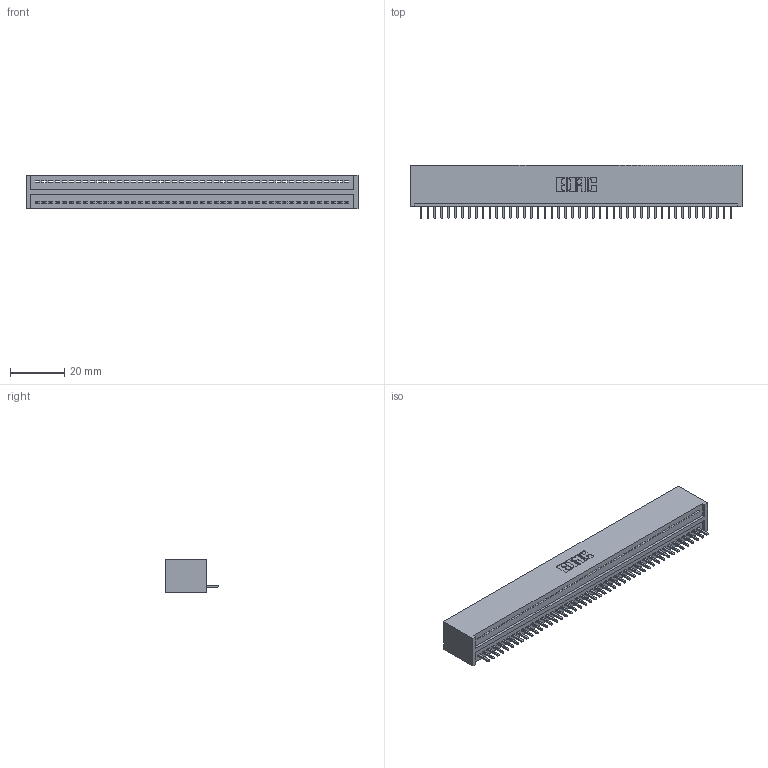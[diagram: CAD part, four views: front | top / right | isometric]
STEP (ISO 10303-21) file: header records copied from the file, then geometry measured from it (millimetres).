
FILE_DESCRIPTION (( 'STEP AP203' ), '1' );
FILE_NAME ('325-046-520-101.STEP', '2020-02-24T22:50:58', ( '' ), ( '' ), 'SwSTEP 2.0', 'SolidWorks 2016', '' );
FILE_SCHEMA (( 'CONFIG_CONTROL_DESIGN' ));
Length unit declared in the file: inch
Products named in the file (3): 325-292-001_325-293-120; 325 Part_Lugless; 325-046-520-101
Assembly tree (47 placements, depth 2):
  325-046-520-101
    325 Part_Lugless
    325-292-001_325-293-120  x46
Bounding box: 122.48 x 19.68 x 12.45 mm (x, y, z)
Volume: 16032.9 mm3; surface area: 17590.6 mm2
Topology: 47 solids, 47 shells, 2774 faces, 8383 edges, 5526 vertices
Faces by surface type: plane 1998, cylinder 776
Entity records: 27345 total; most frequent: CARTESIAN_POINT 4724, ORIENTED_EDGE 4706, DIRECTION 3969, EDGE_CURVE 2353, VECTOR 2233, LINE 2233, VERTEX_POINT 1566, AXIS2_PLACEMENT_3D 868
